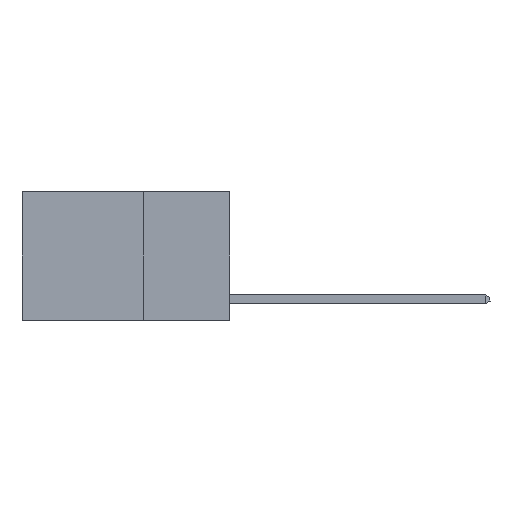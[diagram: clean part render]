
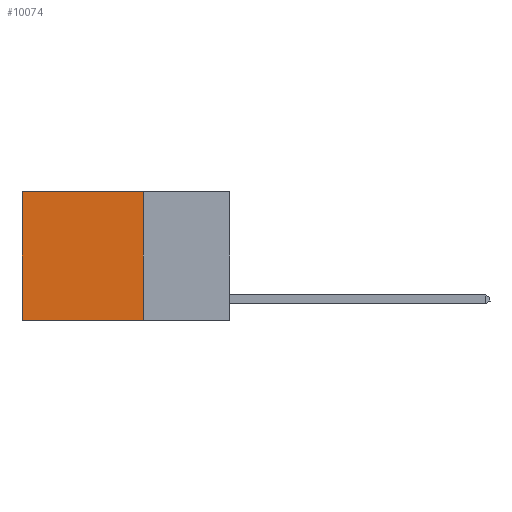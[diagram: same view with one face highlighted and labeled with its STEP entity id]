
A CAD part, left-side view. The second image highlights one B-rep face of the part: STEP entity #10074.
In plain terms, the highlighted planar face has unit normal (-1, 0, 0).
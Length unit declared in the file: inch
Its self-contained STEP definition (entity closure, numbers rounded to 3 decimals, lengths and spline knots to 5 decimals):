
#917 = CARTESIAN_POINT ( 'NONE',  ( 0.2625, 0.25, 0. ) ) ;
#1247 = LINE ( 'NONE', #10381, #5011 ) ;
#2534 = LINE ( 'NONE', #917, #12931 ) ;
#2945 = EDGE_CURVE ( 'NONE', #12415, #5248, #2534, .T. ) ;
#3395 = CARTESIAN_POINT ( 'NONE',  ( 0.2625, 0.25, 0. ) ) ;
#3751 = ORIENTED_EDGE ( 'NONE', *, *, #2945, .F. ) ;
#4510 = DIRECTION ( 'NONE',  ( 0., 1., 0. ) ) ;
#4512 = VECTOR ( 'NONE', #8360, 39.37008 ) ;
#4891 = DIRECTION ( 'NONE',  ( 0., 0., -1. ) ) ;
#5011 = VECTOR ( 'NONE', #4510, 39.37008 ) ;
#5248 = VERTEX_POINT ( 'NONE', #15273 ) ;
#5907 = ORIENTED_EDGE ( 'NONE', *, *, #14116, .T. ) ;
#6229 = CARTESIAN_POINT ( 'NONE',  ( 0.2625, 0.6, 0. ) ) ;
#6244 = DIRECTION ( 'NONE',  ( 0., 0., -1. ) ) ;
#6518 = AXIS2_PLACEMENT_3D ( 'NONE', #3395, #13346, #4891 ) ;
#6693 = CARTESIAN_POINT ( 'NONE',  ( 0.2625, 0.25, 0. ) ) ;
#6924 = VERTEX_POINT ( 'NONE', #6229 ) ;
#8112 = LINE ( 'NONE', #18330, #12970 ) ;
#8156 = EDGE_CURVE ( 'NONE', #12415, #6924, #8112, .T. ) ;
#8360 = DIRECTION ( 'NONE',  ( 0., 0., -1. ) ) ;
#8664 = CARTESIAN_POINT ( 'NONE',  ( 0.2625, 0.6, 0. ) ) ;
#9766 = ORIENTED_EDGE ( 'NONE', *, *, #12608, .F. ) ;
#10074 = ADVANCED_FACE ( 'NONE', ( #15981 ), #10573, .F. ) ;
#10234 = ORIENTED_EDGE ( 'NONE', *, *, #8156, .T. ) ;
#10381 = CARTESIAN_POINT ( 'NONE',  ( 0.2625, 0.25, -0.37 ) ) ;
#10573 = PLANE ( 'NONE',  #6518 ) ;
#11234 = DIRECTION ( 'NONE',  ( 0., 1., 0. ) ) ;
#12020 = LINE ( 'NONE', #8664, #4512 ) ;
#12062 = EDGE_LOOP ( 'NONE', ( #5907, #9766, #3751, #10234 ) ) ;
#12415 = VERTEX_POINT ( 'NONE', #6693 ) ;
#12608 = EDGE_CURVE ( 'NONE', #5248, #17263, #1247, .T. ) ;
#12931 = VECTOR ( 'NONE', #6244, 39.37008 ) ;
#12970 = VECTOR ( 'NONE', #11234, 39.37008 ) ;
#13346 = DIRECTION ( 'NONE',  ( 1., 0., 0. ) ) ;
#14116 = EDGE_CURVE ( 'NONE', #6924, #17263, #12020, .T. ) ;
#15273 = CARTESIAN_POINT ( 'NONE',  ( 0.2625, 0.25, -0.37 ) ) ;
#15981 = FACE_OUTER_BOUND ( 'NONE', #12062, .T. ) ;
#16195 = CARTESIAN_POINT ( 'NONE',  ( 0.2625, 0.6, -0.37 ) ) ;
#17263 = VERTEX_POINT ( 'NONE', #16195 ) ;
#18330 = CARTESIAN_POINT ( 'NONE',  ( 0.2625, 0.25, 0. ) ) ;
